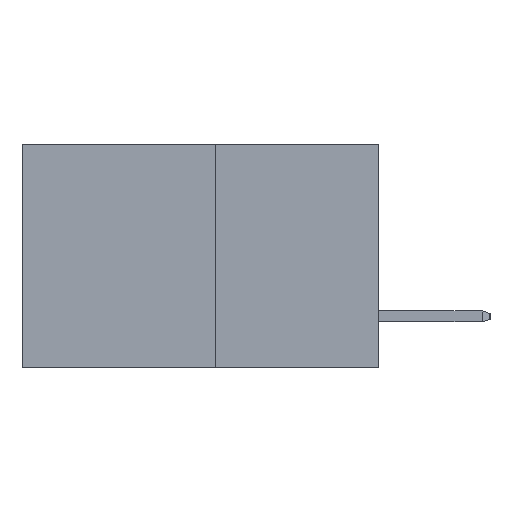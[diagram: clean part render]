
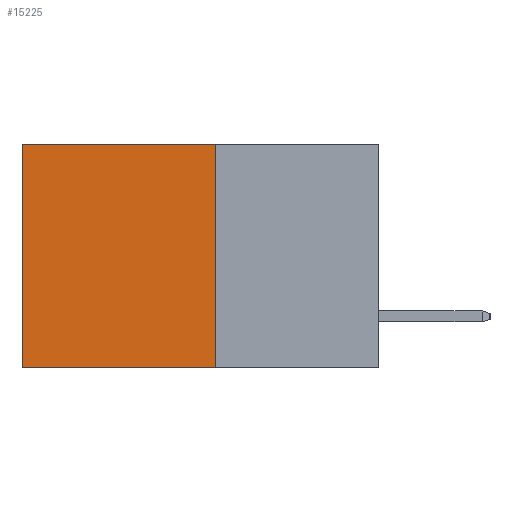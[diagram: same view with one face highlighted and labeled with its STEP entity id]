
A CAD part, left-side view. The second image highlights one B-rep face of the part: STEP entity #15225.
In plain terms, the highlighted planar face has unit normal (-1, 0, 0).
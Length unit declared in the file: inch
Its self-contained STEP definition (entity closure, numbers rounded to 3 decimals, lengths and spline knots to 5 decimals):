
#104 = EDGE_LOOP ( 'NONE', ( #21780, #1891, #22267, #21970 ) ) ;
#1570 = EDGE_CURVE ( 'NONE', #4309, #3542, #18220, .T. ) ;
#1600 = DIRECTION ( 'NONE',  ( 0., 0., -1. ) ) ;
#1891 = ORIENTED_EDGE ( 'NONE', *, *, #31788, .F. ) ;
#2173 = CARTESIAN_POINT ( 'NONE',  ( 0.277, 0.59, 0. ) ) ;
#3269 = LINE ( 'NONE', #12523, #16173 ) ;
#3321 = CARTESIAN_POINT ( 'NONE',  ( 0.277, 0.27, 0. ) ) ;
#3542 = VERTEX_POINT ( 'NONE', #4569 ) ;
#4309 = VERTEX_POINT ( 'NONE', #7817 ) ;
#4569 = CARTESIAN_POINT ( 'NONE',  ( 0.277, 0.27, -0.37 ) ) ;
#7601 = CARTESIAN_POINT ( 'NONE',  ( 0.277, 0.27, -0.37 ) ) ;
#7817 = CARTESIAN_POINT ( 'NONE',  ( 0.277, 0.27, 0. ) ) ;
#10056 = PLANE ( 'NONE',  #19927 ) ;
#10156 = DIRECTION ( 'NONE',  ( 0., 0., -1. ) ) ;
#10568 = CARTESIAN_POINT ( 'NONE',  ( 0.277, 0.27, -0.37 ) ) ;
#11106 = DIRECTION ( 'NONE',  ( 0., 1., 0. ) ) ;
#11195 = VERTEX_POINT ( 'NONE', #2173 ) ;
#12523 = CARTESIAN_POINT ( 'NONE',  ( 0.277, 0.59, -0.37 ) ) ;
#14003 = CARTESIAN_POINT ( 'NONE',  ( 0.277, 0.59, -0.37 ) ) ;
#15225 = ADVANCED_FACE ( 'NONE', ( #26902 ), #10056, .F. ) ;
#16173 = VECTOR ( 'NONE', #32989, 39.37008 ) ;
#16505 = CARTESIAN_POINT ( 'NONE',  ( 0.277, 0.27, -0.37 ) ) ;
#16796 = EDGE_CURVE ( 'NONE', #4309, #11195, #31615, .T. ) ;
#18220 = LINE ( 'NONE', #16505, #31831 ) ;
#18371 = VECTOR ( 'NONE', #31074, 39.37008 ) ;
#19927 = AXIS2_PLACEMENT_3D ( 'NONE', #7601, #25551, #10156 ) ;
#21780 = ORIENTED_EDGE ( 'NONE', *, *, #24202, .T. ) ;
#21970 = ORIENTED_EDGE ( 'NONE', *, *, #16796, .T. ) ;
#22267 = ORIENTED_EDGE ( 'NONE', *, *, #1570, .F. ) ;
#24055 = VECTOR ( 'NONE', #11106, 39.37008 ) ;
#24202 = EDGE_CURVE ( 'NONE', #11195, #31362, #3269, .T. ) ;
#25168 = LINE ( 'NONE', #10568, #18371 ) ;
#25551 = DIRECTION ( 'NONE',  ( 1., 0., 0. ) ) ;
#26902 = FACE_OUTER_BOUND ( 'NONE', #104, .T. ) ;
#31074 = DIRECTION ( 'NONE',  ( 0., 1., 0. ) ) ;
#31362 = VERTEX_POINT ( 'NONE', #14003 ) ;
#31615 = LINE ( 'NONE', #3321, #24055 ) ;
#31788 = EDGE_CURVE ( 'NONE', #3542, #31362, #25168, .T. ) ;
#31831 = VECTOR ( 'NONE', #1600, 39.37008 ) ;
#32989 = DIRECTION ( 'NONE',  ( 0., 0., -1. ) ) ;
